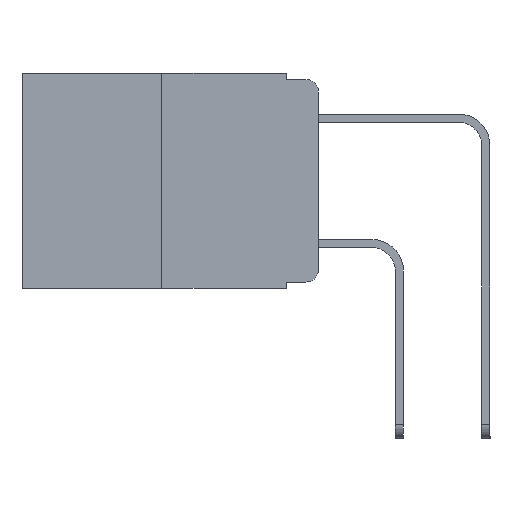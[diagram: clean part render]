
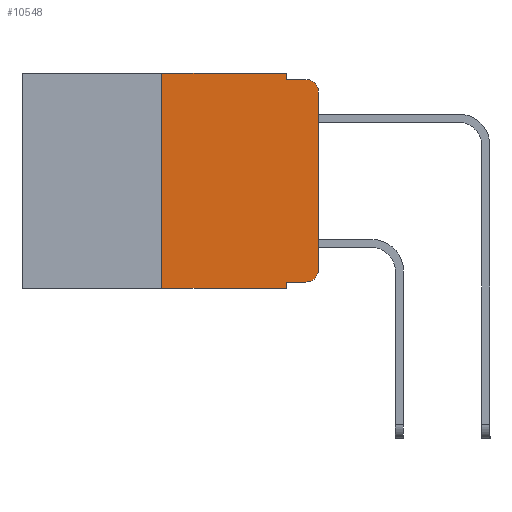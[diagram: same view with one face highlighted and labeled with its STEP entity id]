
A CAD part, left-side view. The second image highlights one B-rep face of the part: STEP entity #10548.
In plain terms, the highlighted planar face has unit normal (-1, 0, 0).
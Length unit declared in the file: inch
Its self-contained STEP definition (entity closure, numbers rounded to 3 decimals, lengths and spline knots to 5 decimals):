
#17 = CARTESIAN_POINT ( 'NONE',  ( 0., 0.473, 0. ) ) ;
#269 = CIRCLE ( 'NONE', #23518, 0.02 ) ;
#635 = AXIS2_PLACEMENT_3D ( 'NONE', #1427, #14878, #3437 ) ;
#734 = EDGE_CURVE ( 'NONE', #770, #830, #6409, .T. ) ;
#770 = VERTEX_POINT ( 'NONE', #17737 ) ;
#830 = VERTEX_POINT ( 'NONE', #11376 ) ;
#1128 = ORIENTED_EDGE ( 'NONE', *, *, #11580, .F. ) ;
#1178 = LINE ( 'NONE', #11875, #15897 ) ;
#1216 = EDGE_CURVE ( 'NONE', #10225, #9894, #1178, .T. ) ;
#1427 = CARTESIAN_POINT ( 'NONE',  ( 0., 0.02, -0.313 ) ) ;
#1451 = VECTOR ( 'NONE', #24016, 39.37008 ) ;
#1508 = CARTESIAN_POINT ( 'NONE',  ( 0., 0., -0.313 ) ) ;
#1750 = EDGE_CURVE ( 'NONE', #830, #17836, #20270, .T. ) ;
#2024 = ORIENTED_EDGE ( 'NONE', *, *, #734, .F. ) ;
#2069 = ORIENTED_EDGE ( 'NONE', *, *, #1216, .F. ) ;
#2592 = VERTEX_POINT ( 'NONE', #7194 ) ;
#2634 = CARTESIAN_POINT ( 'NONE',  ( 0., 0.051, -0.333 ) ) ;
#3094 = CARTESIAN_POINT ( 'NONE',  ( 0., 0.051, -0.343 ) ) ;
#3244 = DIRECTION ( 'NONE',  ( 0., -1., 0. ) ) ;
#3437 = DIRECTION ( 'NONE',  ( 0., 0., -1. ) ) ;
#3457 = VECTOR ( 'NONE', #21517, 39.37008 ) ;
#3814 = EDGE_CURVE ( 'NONE', #13950, #17836, #269, .T. ) ;
#4044 = DIRECTION ( 'NONE',  ( 1., 0., 0. ) ) ;
#4253 = ORIENTED_EDGE ( 'NONE', *, *, #14121, .T. ) ;
#4677 = LINE ( 'NONE', #2634, #3457 ) ;
#4700 = DIRECTION ( 'NONE',  ( 0., -1., 0. ) ) ;
#5652 = ORIENTED_EDGE ( 'NONE', *, *, #3814, .T. ) ;
#6299 = LINE ( 'NONE', #20729, #16422 ) ;
#6362 = ORIENTED_EDGE ( 'NONE', *, *, #10934, .T. ) ;
#6409 = LINE ( 'NONE', #22869, #20875 ) ;
#6547 = CARTESIAN_POINT ( 'NONE',  ( 0., 0.473, 0. ) ) ;
#6682 = ORIENTED_EDGE ( 'NONE', *, *, #13714, .T. ) ;
#7003 = CARTESIAN_POINT ( 'NONE',  ( 0., 0.051, -0.333 ) ) ;
#7194 = CARTESIAN_POINT ( 'NONE',  ( 0., 0.25, -0.343 ) ) ;
#7677 = VERTEX_POINT ( 'NONE', #9838 ) ;
#8525 = EDGE_CURVE ( 'NONE', #7677, #770, #11611, .T. ) ;
#9767 = LINE ( 'NONE', #15425, #14233 ) ;
#9838 = CARTESIAN_POINT ( 'NONE',  ( 0., 0.25, 0. ) ) ;
#9894 = VERTEX_POINT ( 'NONE', #3094 ) ;
#9987 = VECTOR ( 'NONE', #3244, 39.37008 ) ;
#10225 = VERTEX_POINT ( 'NONE', #7003 ) ;
#10548 = ADVANCED_FACE ( 'NONE', ( #21099 ), #15474, .F. ) ;
#10934 = EDGE_CURVE ( 'NONE', #2592, #9894, #12916, .T. ) ;
#11376 = CARTESIAN_POINT ( 'NONE',  ( 0., 0.051, -0.01 ) ) ;
#11534 = CARTESIAN_POINT ( 'NONE',  ( 0., 0.051, -0.01 ) ) ;
#11580 = EDGE_CURVE ( 'NONE', #2592, #7677, #6299, .T. ) ;
#11611 = LINE ( 'NONE', #6547, #20977 ) ;
#11629 = CARTESIAN_POINT ( 'NONE',  ( 0., 0., -0.03 ) ) ;
#11875 = CARTESIAN_POINT ( 'NONE',  ( 0., 0.051, 0. ) ) ;
#12916 = LINE ( 'NONE', #14708, #1451 ) ;
#13509 = DIRECTION ( 'NONE',  ( 0., 0., 1. ) ) ;
#13714 = EDGE_CURVE ( 'NONE', #14753, #15722, #16303, .T. ) ;
#13950 = VERTEX_POINT ( 'NONE', #11629 ) ;
#14121 = EDGE_CURVE ( 'NONE', #10225, #14753, #4677, .T. ) ;
#14230 = DIRECTION ( 'NONE',  ( 0., 0., -1. ) ) ;
#14233 = VECTOR ( 'NONE', #13509, 39.37008 ) ;
#14708 = CARTESIAN_POINT ( 'NONE',  ( 0., 0.473, -0.343 ) ) ;
#14753 = VERTEX_POINT ( 'NONE', #21490 ) ;
#14804 = DIRECTION ( 'NONE',  ( -1., 0., 0. ) ) ;
#14862 = CARTESIAN_POINT ( 'NONE',  ( 0., 0.02, -0.03 ) ) ;
#14878 = DIRECTION ( 'NONE',  ( -1., 0., 0. ) ) ;
#14893 = DIRECTION ( 'NONE',  ( 0., 0., -1. ) ) ;
#15110 = DIRECTION ( 'NONE',  ( 0., 0., 1. ) ) ;
#15425 = CARTESIAN_POINT ( 'NONE',  ( 0., 0., 0. ) ) ;
#15474 = PLANE ( 'NONE',  #17496 ) ;
#15722 = VERTEX_POINT ( 'NONE', #1508 ) ;
#15897 = VECTOR ( 'NONE', #23375, 39.37008 ) ;
#16303 = CIRCLE ( 'NONE', #635, 0.02 ) ;
#16422 = VECTOR ( 'NONE', #15110, 39.37008 ) ;
#17363 = DIRECTION ( 'NONE',  ( 0., 0., -1. ) ) ;
#17496 = AXIS2_PLACEMENT_3D ( 'NONE', #17, #4044, #17363 ) ;
#17737 = CARTESIAN_POINT ( 'NONE',  ( 0., 0.051, 0. ) ) ;
#17836 = VERTEX_POINT ( 'NONE', #24533 ) ;
#18499 = ORIENTED_EDGE ( 'NONE', *, *, #20467, .T. ) ;
#19189 = ORIENTED_EDGE ( 'NONE', *, *, #1750, .F. ) ;
#20270 = LINE ( 'NONE', #11534, #9987 ) ;
#20467 = EDGE_CURVE ( 'NONE', #15722, #13950, #9767, .T. ) ;
#20729 = CARTESIAN_POINT ( 'NONE',  ( 0., 0.25, 0. ) ) ;
#20766 = ORIENTED_EDGE ( 'NONE', *, *, #8525, .F. ) ;
#20875 = VECTOR ( 'NONE', #14893, 39.37008 ) ;
#20977 = VECTOR ( 'NONE', #4700, 39.37008 ) ;
#21099 = FACE_OUTER_BOUND ( 'NONE', #23470, .T. ) ;
#21490 = CARTESIAN_POINT ( 'NONE',  ( 0., 0.02, -0.333 ) ) ;
#21517 = DIRECTION ( 'NONE',  ( 0., -1., 0. ) ) ;
#22869 = CARTESIAN_POINT ( 'NONE',  ( 0., 0.051, 0. ) ) ;
#23375 = DIRECTION ( 'NONE',  ( 0., 0., -1. ) ) ;
#23470 = EDGE_LOOP ( 'NONE', ( #18499, #5652, #19189, #2024, #20766, #1128, #6362, #2069, #4253, #6682 ) ) ;
#23518 = AXIS2_PLACEMENT_3D ( 'NONE', #14862, #14804, #14230 ) ;
#24016 = DIRECTION ( 'NONE',  ( 0., -1., 0. ) ) ;
#24533 = CARTESIAN_POINT ( 'NONE',  ( 0., 0.02, -0.01 ) ) ;
